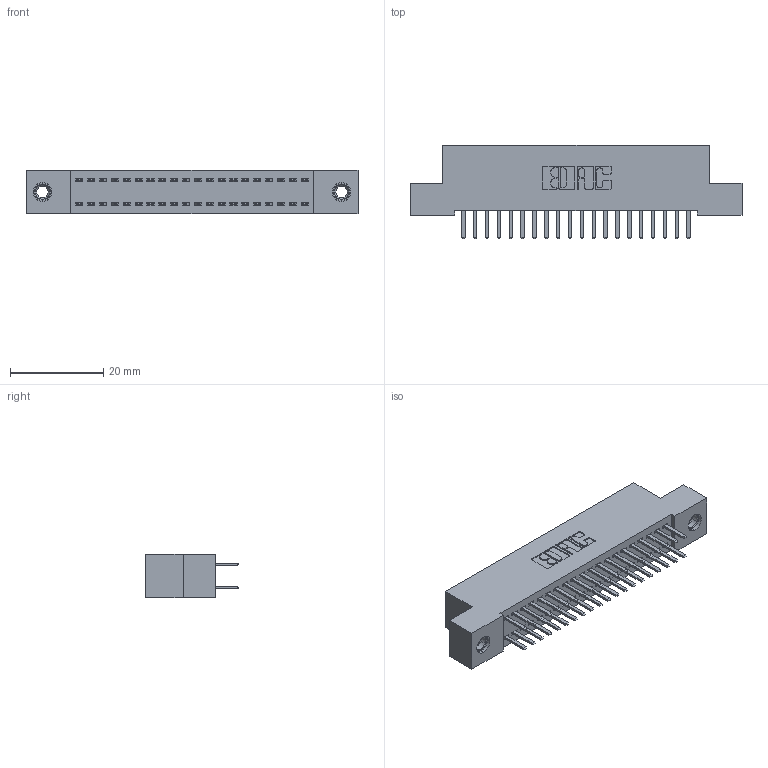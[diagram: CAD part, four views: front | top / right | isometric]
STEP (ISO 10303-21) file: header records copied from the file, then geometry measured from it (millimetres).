
FILE_DESCRIPTION (( 'STEP AP203' ), '1' );
FILE_NAME ('342-040-520-207.STEP', '2019-10-02T15:51:32', ( '' ), ( '' ), 'SwSTEP 2.0', 'SolidWorks 2016', '' );
FILE_SCHEMA (( 'CONFIG_CONTROL_DESIGN' ));
Length unit declared in the file: inch
Products named in the file (4): 345-292-001_345-293-120; 345-250-001_345-250-005-103; 342-040-520-207; 342 Part_TI
Assembly tree (43 placements, depth 2):
  342-040-520-207
    342 Part_TI
    345-292-001_345-293-120  x40
    345-250-001_345-250-005-103  x2
Bounding box: 71.12 x 20.02 x 9.4 mm (x, y, z)
Volume: 6255.7 mm3; surface area: 9624.9 mm2
Topology: 43 solids, 43 shells, 2410 faces, 6955 edges, 4522 vertices
Faces by surface type: plane 1618, cylinder 776, cone 12, torus 4
Entity records: 16880 total; most frequent: CARTESIAN_POINT 2817, ORIENTED_EDGE 2734, DIRECTION 2465, EDGE_CURVE 1367, LINE 1215, VECTOR 1215, VERTEX_POINT 904, AXIS2_PLACEMENT_3D 625
